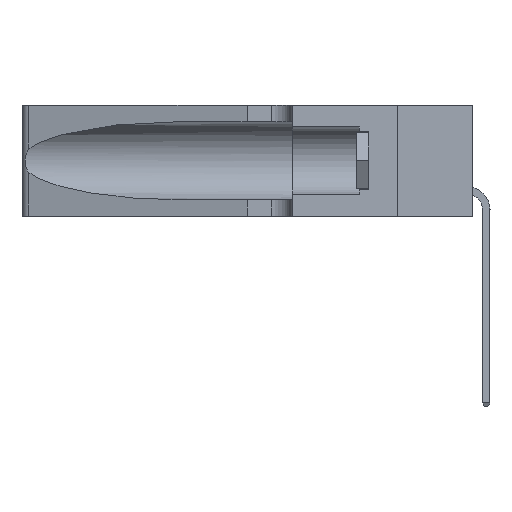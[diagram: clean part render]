
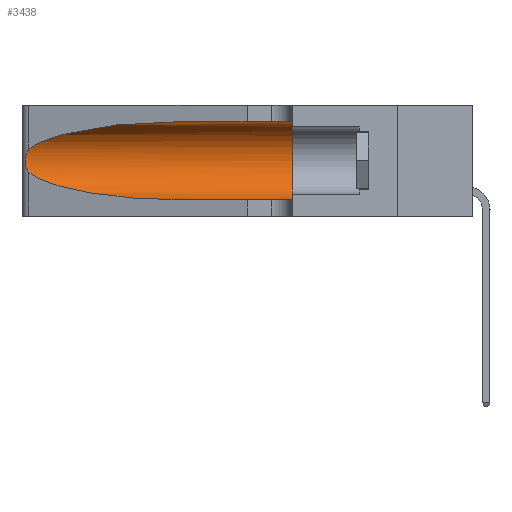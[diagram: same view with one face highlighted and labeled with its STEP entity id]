
A CAD part, left-side view. The second image highlights one B-rep face of the part: STEP entity #3438.
In plain terms, the highlighted cylindrical face has radius 3.308 mm (diameter 6.617 mm), a partial arc.
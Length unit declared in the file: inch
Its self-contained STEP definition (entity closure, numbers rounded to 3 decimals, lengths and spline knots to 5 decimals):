
#346 = VERTEX_POINT ( 'NONE', #33565 ) ;
#2178 = CARTESIAN_POINT ( 'NONE',  ( 0.26017, 1.23833, 0.17102 ) ) ;
#2277 = VECTOR ( 'NONE', #30900, 39.37008 ) ;
#2457 = CARTESIAN_POINT ( 'NONE',  ( 0.25555, 1.22993, 0.14849 ) ) ;
#2512 = CARTESIAN_POINT ( 'NONE',  ( 0.25487, 1.22718, 0.14631 ) ) ;
#3438 = ADVANCED_FACE ( 'NONE', ( #5281 ), #31825, .F. ) ;
#3523 = VERTEX_POINT ( 'NONE', #25561 ) ;
#3895 = DIRECTION ( 'NONE',  ( 0., 0., 1. ) ) ;
#4088 = DIRECTION ( 'NONE',  ( 0., -1., 0. ) ) ;
#5281 = FACE_OUTER_BOUND ( 'NONE', #23328, .T. ) ;
#5339 = CARTESIAN_POINT ( 'NONE',  ( 0.25856, 1.23593, 0.16098 ) ) ;
#5452 = CARTESIAN_POINT ( 'NONE',  ( 0.25487, 1.22718, 0.22369 ) ) ;
#7485 = CARTESIAN_POINT ( 'NONE',  ( 0.1305, 1.61858, 0.05475 ) ) ;
#9607 = ORIENTED_EDGE ( 'NONE', *, *, #31712, .F. ) ;
#9976 = ORIENTED_EDGE ( 'NONE', *, *, #32181, .F. ) ;
#10505 = CARTESIAN_POINT ( 'NONE',  ( 0.26075, 1.23896, 0.178 ) ) ;
#12413 = B_SPLINE_CURVE_WITH_KNOTS ( 'NONE', 3,
 ( #5452, #28248, #31241, #28892, #16445, #30657, #13785, #10505, #2178, #5339, #22204, #32385, #2457, #32255 ),
 .UNSPECIFIED., .F., .F.,
 ( 4, 2, 2, 2, 2, 2, 4 ),
 ( 0., 0.00027, 0.00053, 0.00107, 0.0016, 0.00187, 0.00214 ),
 .UNSPECIFIED. ) ;
#13625 = CARTESIAN_POINT ( 'NONE',  ( 0.2373, 1.15595, 0.08982 ) ) ;
#13785 = CARTESIAN_POINT ( 'NONE',  ( 0.26075, 1.23896, 0.19203 ) ) ;
#14137 = CARTESIAN_POINT ( 'NONE',  ( 0.25487, 1.22718, 0.22369 ) ) ;
#15571 = EDGE_CURVE ( 'NONE', #19037, #26885, #12413, .T. ) ;
#15639 = VERTEX_POINT ( 'NONE', #35884 ) ;
#16204 = CARTESIAN_POINT ( 'NONE',  ( 0.1305, 0.35, 0.185 ) ) ;
#16445 = CARTESIAN_POINT ( 'NONE',  ( 0.25854, 1.2359, 0.20912 ) ) ;
#17940 = VECTOR ( 'NONE', #4088, 39.37008 ) ;
#19001 = DIRECTION ( 'NONE',  ( 0., -1., 0. ) ) ;
#19037 = VERTEX_POINT ( 'NONE', #34636 ) ;
#19387 = EDGE_CURVE ( 'NONE', #33337, #15639, #30845, .T. ) ;
#19655 =( BOUNDED_CURVE ( )  B_SPLINE_CURVE ( 3, ( #37401, #37253, #37102, #14137 ),
 .UNSPECIFIED., .F., .F. ) 
 B_SPLINE_CURVE_WITH_KNOTS ( ( 4, 4 ),
 ( 1.5708, 2.84003 ),
 .UNSPECIFIED. ) 
 CURVE ( )  GEOMETRIC_REPRESENTATION_ITEM ( )  RATIONAL_B_SPLINE_CURVE ( ( 1., 0.87, 0.87, 1. ) ) 
 REPRESENTATION_ITEM ( '' )  );
#21709 = ORIENTED_EDGE ( 'NONE', *, *, #23867, .T. ) ;
#22204 = CARTESIAN_POINT ( 'NONE',  ( 0.25789, 1.23486, 0.15765 ) ) ;
#22959 = CIRCLE ( 'NONE', #30255, 0.13025 ) ;
#23328 = EDGE_LOOP ( 'NONE', ( #21709, #42323, #40352, #30581, #9976, #9607 ) ) ;
#23867 = EDGE_CURVE ( 'NONE', #3523, #19037, #19655, .T. ) ;
#25037 = CARTESIAN_POINT ( 'NONE',  ( 0.25487, 1.22718, 0.14631 ) ) ;
#25561 = CARTESIAN_POINT ( 'NONE',  ( 0.1305, 0.72297, 0.31525 ) ) ;
#26885 = VERTEX_POINT ( 'NONE', #2512 ) ;
#28248 = CARTESIAN_POINT ( 'NONE',  ( 0.25555, 1.22994, 0.2215 ) ) ;
#28892 = CARTESIAN_POINT ( 'NONE',  ( 0.25787, 1.23484, 0.2124 ) ) ;
#29252 =( BOUNDED_CURVE ( )  B_SPLINE_CURVE ( 3, ( #25037, #13625, #36767, #39113 ),
 .UNSPECIFIED., .F., .F. ) 
 B_SPLINE_CURVE_WITH_KNOTS ( ( 4, 4 ),
 ( 3.44316, 4.71239 ),
 .UNSPECIFIED. ) 
 CURVE ( )  GEOMETRIC_REPRESENTATION_ITEM ( )  RATIONAL_B_SPLINE_CURVE ( ( 1., 0.87, 0.87, 1. ) ) 
 REPRESENTATION_ITEM ( '' )  );
#29449 = EDGE_CURVE ( 'NONE', #26885, #33337, #29252, .T. ) ;
#30255 = AXIS2_PLACEMENT_3D ( 'NONE', #16204, #32897, #3895 ) ;
#30581 = ORIENTED_EDGE ( 'NONE', *, *, #19387, .T. ) ;
#30657 = CARTESIAN_POINT ( 'NONE',  ( 0.26018, 1.23835, 0.19895 ) ) ;
#30845 = LINE ( 'NONE', #7485, #2277 ) ;
#30900 = DIRECTION ( 'NONE',  ( 0., -1., 0. ) ) ;
#31241 = CARTESIAN_POINT ( 'NONE',  ( 0.25639, 1.23184, 0.21858 ) ) ;
#31712 = EDGE_CURVE ( 'NONE', #3523, #346, #40294, .T. ) ;
#31825 = CYLINDRICAL_SURFACE ( 'NONE', #43091, 0.13025 ) ;
#32079 = CARTESIAN_POINT ( 'NONE',  ( 0.1305, 1.61858, 0.185 ) ) ;
#32181 = EDGE_CURVE ( 'NONE', #346, #15639, #22959, .T. ) ;
#32255 = CARTESIAN_POINT ( 'NONE',  ( 0.25487, 1.22718, 0.14631 ) ) ;
#32362 = DIRECTION ( 'NONE',  ( 0., 0., -1. ) ) ;
#32385 = CARTESIAN_POINT ( 'NONE',  ( 0.25639, 1.23186, 0.15144 ) ) ;
#32897 = DIRECTION ( 'NONE',  ( 0., 1., 0. ) ) ;
#33337 = VERTEX_POINT ( 'NONE', #36448 ) ;
#33565 = CARTESIAN_POINT ( 'NONE',  ( 0.1305, 0.35, 0.31525 ) ) ;
#33909 = CARTESIAN_POINT ( 'NONE',  ( 0.1305, 1.61858, 0.31525 ) ) ;
#34636 = CARTESIAN_POINT ( 'NONE',  ( 0.25487, 1.22718, 0.22369 ) ) ;
#35884 = CARTESIAN_POINT ( 'NONE',  ( 0.1305, 0.35, 0.05475 ) ) ;
#36448 = CARTESIAN_POINT ( 'NONE',  ( 0.1305, 0.72297, 0.05475 ) ) ;
#36767 = CARTESIAN_POINT ( 'NONE',  ( 0.18966, 0.96281, 0.05475 ) ) ;
#37102 = CARTESIAN_POINT ( 'NONE',  ( 0.2373, 1.15595, 0.28018 ) ) ;
#37253 = CARTESIAN_POINT ( 'NONE',  ( 0.18966, 0.96281, 0.31525 ) ) ;
#37401 = CARTESIAN_POINT ( 'NONE',  ( 0.1305, 0.72297, 0.31525 ) ) ;
#39113 = CARTESIAN_POINT ( 'NONE',  ( 0.1305, 0.72297, 0.05475 ) ) ;
#40294 = LINE ( 'NONE', #33909, #17940 ) ;
#40352 = ORIENTED_EDGE ( 'NONE', *, *, #29449, .T. ) ;
#42323 = ORIENTED_EDGE ( 'NONE', *, *, #15571, .T. ) ;
#43091 = AXIS2_PLACEMENT_3D ( 'NONE', #32079, #19001, #32362 ) ;
